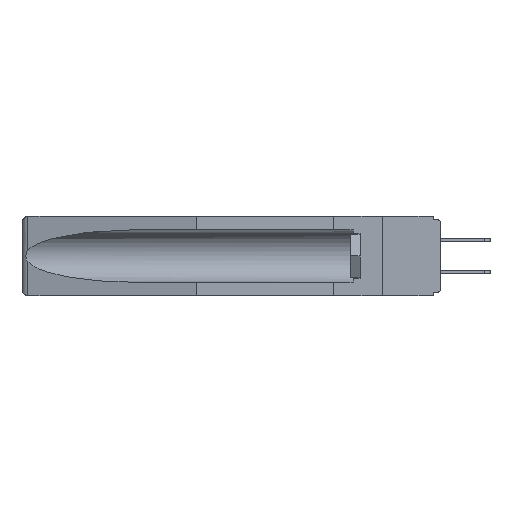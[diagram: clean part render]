
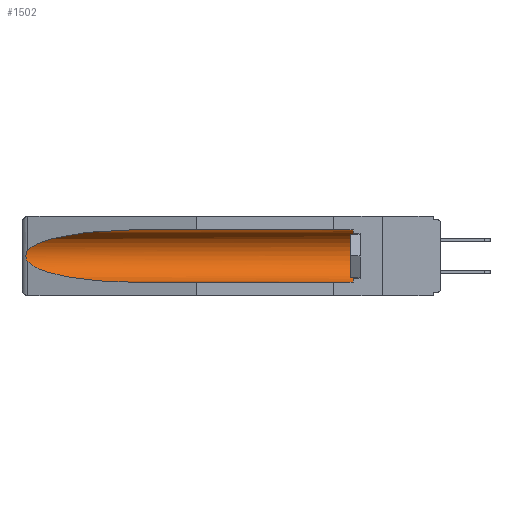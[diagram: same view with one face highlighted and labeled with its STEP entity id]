
A CAD part, left-side view. The second image highlights one B-rep face of the part: STEP entity #1502.
In plain terms, the highlighted cylindrical face has radius 2.857 mm (diameter 5.715 mm), a partial arc.
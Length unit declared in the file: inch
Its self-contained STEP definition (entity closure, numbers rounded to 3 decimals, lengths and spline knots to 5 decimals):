
#460 = CARTESIAN_POINT ( 'NONE',  ( 0.25451, 1.48313, -0.09465 ) ) ;
#913 = CARTESIAN_POINT ( 'NONE',  ( 0.155, 1.07973, -0.284 ) ) ;
#1193 = ORIENTED_EDGE ( 'NONE', *, *, #13601, .T. ) ;
#1438 = DIRECTION ( 'NONE',  ( 0., 0., 1. ) ) ;
#1502 = ADVANCED_FACE ( 'NONE', ( #8515 ), #1710, .F. ) ;
#1648 = B_SPLINE_CURVE_WITH_KNOTS ( 'NONE', 3,
 ( #18375, #9183, #12270, #13836, #2106, #18239, #12148, #4356, #6142, #10659 ),
 .UNSPECIFIED., .F., .F.,
 ( 4, 2, 2, 2, 4 ),
 ( 0., 0.00029, 0.00058, 0.00087, 0.00117 ),
 .UNSPECIFIED. ) ;
#1710 = CYLINDRICAL_SURFACE ( 'NONE', #14688, 0.1125 ) ;
#2106 = CARTESIAN_POINT ( 'NONE',  ( 0.2675, 1.53308, -0.16763 ) ) ;
#2994 = DIRECTION ( 'NONE',  ( 0., 1., 0. ) ) ;
#3201 = ORIENTED_EDGE ( 'NONE', *, *, #15215, .T. ) ;
#3219 = ORIENTED_EDGE ( 'NONE', *, *, #6686, .T. ) ;
#3488 = VERTEX_POINT ( 'NONE', #10884 ) ;
#3858 = DIRECTION ( 'NONE',  ( 0., 1., 0. ) ) ;
#4356 = CARTESIAN_POINT ( 'NONE',  ( 0.26655, 1.53094, -0.18657 ) ) ;
#4421 = EDGE_CURVE ( 'NONE', #3488, #15021, #6957, .T. ) ;
#5996 = CARTESIAN_POINT ( 'NONE',  ( 0.155, -0.30754, -0.1715 ) ) ;
#6112 = CIRCLE ( 'NONE', #13500, 0.1125 ) ;
#6142 = CARTESIAN_POINT ( 'NONE',  ( 0.26597, 1.5296, -0.19026 ) ) ;
#6350 = CARTESIAN_POINT ( 'NONE',  ( 0.155, 1.07973, -0.059 ) ) ;
#6686 = EDGE_CURVE ( 'NONE', #12835, #17269, #1648, .T. ) ;
#6957 = LINE ( 'NONE', #19734, #8418 ) ;
#6971 = VERTEX_POINT ( 'NONE', #11241 ) ;
#7137 = CARTESIAN_POINT ( 'NONE',  ( 0.26537, 1.52718, -0.19328 ) ) ;
#7141 = ORIENTED_EDGE ( 'NONE', *, *, #10165, .F. ) ;
#7212 = LINE ( 'NONE', #13115, #16577 ) ;
#7268 = CARTESIAN_POINT ( 'NONE',  ( 0.25451, 1.48313, -0.24835 ) ) ;
#7549 = DIRECTION ( 'NONE',  ( 0., 0., 1. ) ) ;
#8172 = EDGE_CURVE ( 'NONE', #17269, #10443, #14525, .T. ) ;
#8418 = VECTOR ( 'NONE', #19664, 39.37008 ) ;
#8515 = FACE_OUTER_BOUND ( 'NONE', #18548, .T. ) ;
#8612 =( BOUNDED_CURVE ( )  B_SPLINE_CURVE ( 3, ( #12762, #18928, #460, #12894 ),
 .UNSPECIFIED., .F., .F. ) 
 B_SPLINE_CURVE_WITH_KNOTS ( ( 4, 4 ),
 ( 4.71239, 6.08839 ),
 .UNSPECIFIED. ) 
 CURVE ( )  GEOMETRIC_REPRESENTATION_ITEM ( )  RATIONAL_B_SPLINE_CURVE ( ( 1., 0.848, 0.848, 1. ) ) 
 REPRESENTATION_ITEM ( '' )  );
#8887 = CARTESIAN_POINT ( 'NONE',  ( 0.21114, 1.30732, -0.284 ) ) ;
#9183 = CARTESIAN_POINT ( 'NONE',  ( 0.26597, 1.52961, -0.15275 ) ) ;
#9445 = CARTESIAN_POINT ( 'NONE',  ( 0.155, 1.07973, -0.284 ) ) ;
#10165 = EDGE_CURVE ( 'NONE', #6971, #10443, #7212, .T. ) ;
#10293 = ORIENTED_EDGE ( 'NONE', *, *, #4421, .T. ) ;
#10443 = VERTEX_POINT ( 'NONE', #9445 ) ;
#10641 = DIRECTION ( 'NONE',  ( 0., -1., 0. ) ) ;
#10659 = CARTESIAN_POINT ( 'NONE',  ( 0.26537, 1.52718, -0.19328 ) ) ;
#10884 = CARTESIAN_POINT ( 'NONE',  ( 0.155, 0.126, -0.059 ) ) ;
#11120 = CARTESIAN_POINT ( 'NONE',  ( 0.26537, 1.52718, -0.14972 ) ) ;
#11241 = CARTESIAN_POINT ( 'NONE',  ( 0.155, 0.126, -0.284 ) ) ;
#12148 = CARTESIAN_POINT ( 'NONE',  ( 0.2673, 1.53269, -0.17917 ) ) ;
#12270 = CARTESIAN_POINT ( 'NONE',  ( 0.26654, 1.53092, -0.15636 ) ) ;
#12313 = CARTESIAN_POINT ( 'NONE',  ( 0.155, 0.126, -0.1715 ) ) ;
#12762 = CARTESIAN_POINT ( 'NONE',  ( 0.155, 1.07973, -0.059 ) ) ;
#12835 = VERTEX_POINT ( 'NONE', #11120 ) ;
#12894 = CARTESIAN_POINT ( 'NONE',  ( 0.26537, 1.52718, -0.14972 ) ) ;
#13115 = CARTESIAN_POINT ( 'NONE',  ( 0.155, -0.30754, -0.284 ) ) ;
#13500 = AXIS2_PLACEMENT_3D ( 'NONE', #12313, #10641, #1438 ) ;
#13601 = EDGE_CURVE ( 'NONE', #6971, #3488, #6112, .T. ) ;
#13836 = CARTESIAN_POINT ( 'NONE',  ( 0.2673, 1.5327, -0.16383 ) ) ;
#14525 =( BOUNDED_CURVE ( )  B_SPLINE_CURVE ( 3, ( #7137, #7268, #8887, #913 ),
 .UNSPECIFIED., .F., .F. ) 
 B_SPLINE_CURVE_WITH_KNOTS ( ( 4, 4 ),
 ( 0.1948, 1.5708 ),
 .UNSPECIFIED. ) 
 CURVE ( )  GEOMETRIC_REPRESENTATION_ITEM ( )  RATIONAL_B_SPLINE_CURVE ( ( 1., 0.848, 0.848, 1. ) ) 
 REPRESENTATION_ITEM ( '' )  );
#14538 = ORIENTED_EDGE ( 'NONE', *, *, #8172, .T. ) ;
#14688 = AXIS2_PLACEMENT_3D ( 'NONE', #5996, #2994, #7549 ) ;
#15021 = VERTEX_POINT ( 'NONE', #6350 ) ;
#15215 = EDGE_CURVE ( 'NONE', #15021, #12835, #8612, .T. ) ;
#15917 = CARTESIAN_POINT ( 'NONE',  ( 0.26537, 1.52718, -0.19328 ) ) ;
#16577 = VECTOR ( 'NONE', #3858, 39.37008 ) ;
#17269 = VERTEX_POINT ( 'NONE', #15917 ) ;
#18239 = CARTESIAN_POINT ( 'NONE',  ( 0.2675, 1.53308, -0.17534 ) ) ;
#18375 = CARTESIAN_POINT ( 'NONE',  ( 0.26537, 1.52718, -0.14972 ) ) ;
#18548 = EDGE_LOOP ( 'NONE', ( #3201, #3219, #14538, #7141, #1193, #10293 ) ) ;
#18928 = CARTESIAN_POINT ( 'NONE',  ( 0.21114, 1.30732, -0.059 ) ) ;
#19664 = DIRECTION ( 'NONE',  ( 0., 1., 0. ) ) ;
#19734 = CARTESIAN_POINT ( 'NONE',  ( 0.155, -0.30754, -0.059 ) ) ;
